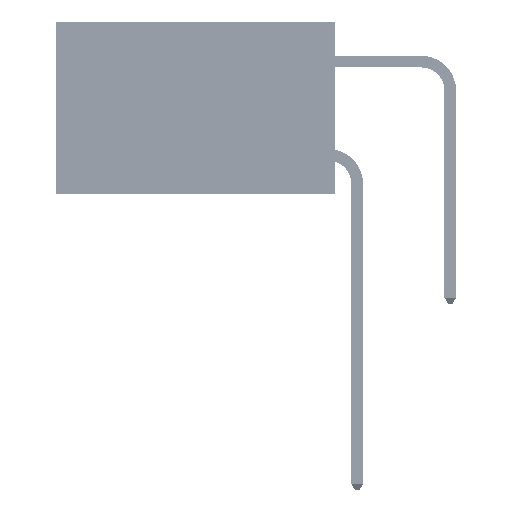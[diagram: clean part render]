
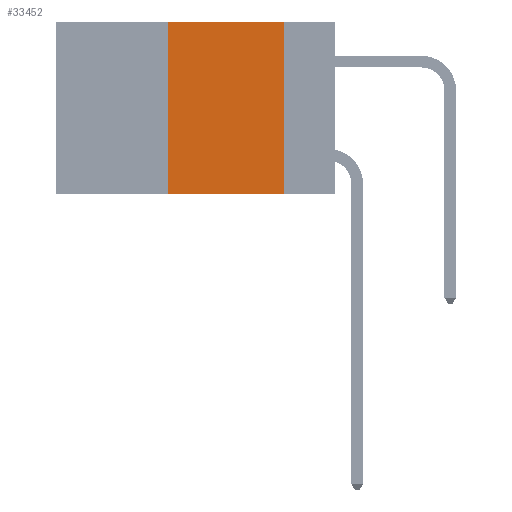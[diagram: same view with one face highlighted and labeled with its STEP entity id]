
A CAD part, left-side view. The second image highlights one B-rep face of the part: STEP entity #33452.
In plain terms, the highlighted planar face has unit normal (-1, 0, 0).
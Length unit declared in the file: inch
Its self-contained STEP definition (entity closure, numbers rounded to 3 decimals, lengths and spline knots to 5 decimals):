
#2087 = LINE ( 'NONE', #16575, #19967 ) ;
#2712 = CARTESIAN_POINT ( 'NONE',  ( 0., 0.11, 0. ) ) ;
#4908 = VERTEX_POINT ( 'NONE', #22364 ) ;
#5852 = ORIENTED_EDGE ( 'NONE', *, *, #17708, .F. ) ;
#5994 = CARTESIAN_POINT ( 'NONE',  ( 0., 0.6, 0. ) ) ;
#10785 = LINE ( 'NONE', #39742, #29263 ) ;
#14039 = CARTESIAN_POINT ( 'NONE',  ( 0., 0.6, -0.37 ) ) ;
#14155 = ORIENTED_EDGE ( 'NONE', *, *, #44163, .F. ) ;
#16575 = CARTESIAN_POINT ( 'NONE',  ( 0., 0.36, 0. ) ) ;
#16703 = CARTESIAN_POINT ( 'NONE',  ( 0., 0.11, 0. ) ) ;
#17708 = EDGE_CURVE ( 'NONE', #38799, #30650, #20262, .T. ) ;
#19967 = VECTOR ( 'NONE', #30811, 39.37008 ) ;
#20262 = LINE ( 'NONE', #16703, #33862 ) ;
#22364 = CARTESIAN_POINT ( 'NONE',  ( 0., 0.36, 0. ) ) ;
#24623 = CARTESIAN_POINT ( 'NONE',  ( 0., 0.11, -0.37 ) ) ;
#27125 = FACE_OUTER_BOUND ( 'NONE', #37011, .T. ) ;
#28055 = DIRECTION ( 'NONE',  ( 0., -1., 0. ) ) ;
#29263 = VECTOR ( 'NONE', #39285, 39.37008 ) ;
#30650 = VERTEX_POINT ( 'NONE', #24623 ) ;
#30811 = DIRECTION ( 'NONE',  ( 0., 0., 1. ) ) ;
#31151 = AXIS2_PLACEMENT_3D ( 'NONE', #5994, #38523, #34725 ) ;
#33452 = ADVANCED_FACE ( 'NONE', ( #27125 ), #42071, .F. ) ;
#33862 = VECTOR ( 'NONE', #34983, 39.37008 ) ;
#34725 = DIRECTION ( 'NONE',  ( 0., 0., -1. ) ) ;
#34983 = DIRECTION ( 'NONE',  ( 0., 0., -1. ) ) ;
#35718 = EDGE_CURVE ( 'NONE', #36066, #4908, #2087, .T. ) ;
#36066 = VERTEX_POINT ( 'NONE', #44260 ) ;
#36546 = ORIENTED_EDGE ( 'NONE', *, *, #35718, .F. ) ;
#37011 = EDGE_LOOP ( 'NONE', ( #5852, #14155, #36546, #42327 ) ) ;
#38261 = VECTOR ( 'NONE', #28055, 39.37008 ) ;
#38519 = LINE ( 'NONE', #14039, #38261 ) ;
#38523 = DIRECTION ( 'NONE',  ( 1., 0., 0. ) ) ;
#38799 = VERTEX_POINT ( 'NONE', #2712 ) ;
#39285 = DIRECTION ( 'NONE',  ( 0., -1., 0. ) ) ;
#39304 = EDGE_CURVE ( 'NONE', #36066, #30650, #38519, .T. ) ;
#39742 = CARTESIAN_POINT ( 'NONE',  ( 0., 0.6, 0. ) ) ;
#42071 = PLANE ( 'NONE',  #31151 ) ;
#42327 = ORIENTED_EDGE ( 'NONE', *, *, #39304, .T. ) ;
#44163 = EDGE_CURVE ( 'NONE', #4908, #38799, #10785, .T. ) ;
#44260 = CARTESIAN_POINT ( 'NONE',  ( 0., 0.36, -0.37 ) ) ;
